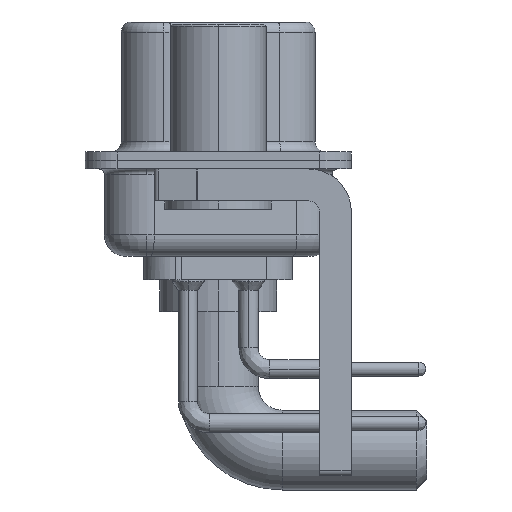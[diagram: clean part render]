
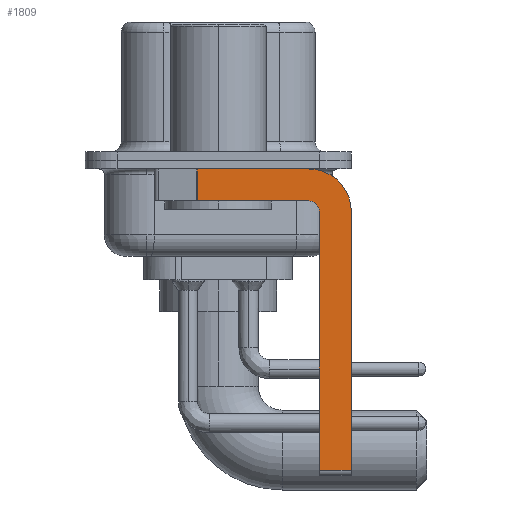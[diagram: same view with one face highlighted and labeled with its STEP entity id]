
A CAD part, left-side view. The second image highlights one B-rep face of the part: STEP entity #1809.
In plain terms, the highlighted planar face has unit normal (-1, 0, 0).
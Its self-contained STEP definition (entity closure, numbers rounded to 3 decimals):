
#289 = VERTEX_POINT ( 'NONE', #27104 ) ;
#622 = VECTOR ( 'NONE', #12479, 1000. ) ;
#795 = VERTEX_POINT ( 'NONE', #12686 ) ;
#1060 = AXIS2_PLACEMENT_3D ( 'NONE', #16492, #27981, #20971 ) ;
#1572 = FACE_OUTER_BOUND ( 'NONE', #23255, .T. ) ;
#1809 = ADVANCED_FACE ( 'NONE', ( #1572 ), #20848, .F. ) ;
#2685 = AXIS2_PLACEMENT_3D ( 'NONE', #13749, #20355, #11168 ) ;
#2969 = EDGE_CURVE ( 'NONE', #4347, #5563, #23773, .T. ) ;
#3414 = VERTEX_POINT ( 'NONE', #17682 ) ;
#3593 = CARTESIAN_POINT ( 'NONE',  ( -2.9, -4.25, -0.4 ) ) ;
#4347 = VERTEX_POINT ( 'NONE', #28086 ) ;
#5406 = CARTESIAN_POINT ( 'NONE',  ( -2.9, -4.75, -14.8 ) ) ;
#5563 = VERTEX_POINT ( 'NONE', #19250 ) ;
#5698 = CARTESIAN_POINT ( 'NONE',  ( -2.9, -4.25, -1.9 ) ) ;
#6378 = LINE ( 'NONE', #10550, #23307 ) ;
#6904 = CARTESIAN_POINT ( 'NONE',  ( -2.9, -4.25, -1.9 ) ) ;
#7136 = EDGE_CURVE ( 'NONE', #10527, #289, #20111, .T. ) ;
#7400 = AXIS2_PLACEMENT_3D ( 'NONE', #25423, #16377, #23000 ) ;
#7750 = LINE ( 'NONE', #18804, #622 ) ;
#8350 = DIRECTION ( 'NONE',  ( 0., -1., 0. ) ) ;
#8371 = ORIENTED_EDGE ( 'NONE', *, *, #26813, .T. ) ;
#9350 = DIRECTION ( 'NONE',  ( 0., 1., 0. ) ) ;
#10527 = VERTEX_POINT ( 'NONE', #5698 ) ;
#10550 = CARTESIAN_POINT ( 'NONE',  ( -2.9, 0.978, -1.9 ) ) ;
#11168 = DIRECTION ( 'NONE',  ( 0., 0., 1. ) ) ;
#11460 = ORIENTED_EDGE ( 'NONE', *, *, #11891, .F. ) ;
#11857 = EDGE_CURVE ( 'NONE', #21754, #4347, #20358, .T. ) ;
#11891 = EDGE_CURVE ( 'NONE', #3414, #21754, #7750, .T. ) ;
#12121 = VECTOR ( 'NONE', #8350, 1000. ) ;
#12479 = DIRECTION ( 'NONE',  ( 0., -1., 0. ) ) ;
#12640 = VECTOR ( 'NONE', #16039, 1000. ) ;
#12686 = CARTESIAN_POINT ( 'NONE',  ( -2.9, -4.75, -2.4 ) ) ;
#12715 = EDGE_CURVE ( 'NONE', #25160, #5563, #14804, .T. ) ;
#12758 = ORIENTED_EDGE ( 'NONE', *, *, #18714, .F. ) ;
#12789 = CARTESIAN_POINT ( 'NONE',  ( -2.9, -4.25, -14.55 ) ) ;
#13749 = CARTESIAN_POINT ( 'NONE',  ( -2.9, -4.25, -2.4 ) ) ;
#14804 = LINE ( 'NONE', #12789, #12121 ) ;
#14861 = DIRECTION ( 'NONE',  ( 0., 0., -1. ) ) ;
#15983 = CIRCLE ( 'NONE', #2685, 0.5 ) ;
#16039 = DIRECTION ( 'NONE',  ( 0., 0., 1. ) ) ;
#16377 = DIRECTION ( 'NONE',  ( 1., 0., 0. ) ) ;
#16492 = CARTESIAN_POINT ( 'NONE',  ( -2.9, -4.25, -2.4 ) ) ;
#17517 = VECTOR ( 'NONE', #21772, 1000. ) ;
#17682 = CARTESIAN_POINT ( 'NONE',  ( -2.9, 0.978, -0.4 ) ) ;
#17866 = ORIENTED_EDGE ( 'NONE', *, *, #11857, .F. ) ;
#18714 = EDGE_CURVE ( 'NONE', #25160, #795, #25075, .T. ) ;
#18804 = CARTESIAN_POINT ( 'NONE',  ( -2.9, 3., -0.4 ) ) ;
#19250 = CARTESIAN_POINT ( 'NONE',  ( -2.9, -6.25, -14.55 ) ) ;
#19622 = CARTESIAN_POINT ( 'NONE',  ( -2.9, -6.25, -2.4 ) ) ;
#20111 = LINE ( 'NONE', #6904, #23884 ) ;
#20237 = CARTESIAN_POINT ( 'NONE',  ( -2.9, -4.75, -14.55 ) ) ;
#20355 = DIRECTION ( 'NONE',  ( -1., 0., 0. ) ) ;
#20358 = CIRCLE ( 'NONE', #1060, 2. ) ;
#20848 = PLANE ( 'NONE',  #7400 ) ;
#20971 = DIRECTION ( 'NONE',  ( 0., 0., -1. ) ) ;
#21754 = VERTEX_POINT ( 'NONE', #3593 ) ;
#21772 = DIRECTION ( 'NONE',  ( 0., 0., -1. ) ) ;
#22772 = ORIENTED_EDGE ( 'NONE', *, *, #27979, .F. ) ;
#23000 = DIRECTION ( 'NONE',  ( 0., 0., -1. ) ) ;
#23255 = EDGE_LOOP ( 'NONE', ( #11460, #8371, #26242, #22772, #12758, #25396, #27537, #17866 ) ) ;
#23307 = VECTOR ( 'NONE', #14861, 1000. ) ;
#23773 = LINE ( 'NONE', #19622, #17517 ) ;
#23884 = VECTOR ( 'NONE', #9350, 1000. ) ;
#25075 = LINE ( 'NONE', #5406, #12640 ) ;
#25160 = VERTEX_POINT ( 'NONE', #20237 ) ;
#25396 = ORIENTED_EDGE ( 'NONE', *, *, #12715, .T. ) ;
#25423 = CARTESIAN_POINT ( 'NONE',  ( -2.9, -4.25, -2.4 ) ) ;
#26242 = ORIENTED_EDGE ( 'NONE', *, *, #7136, .F. ) ;
#26813 = EDGE_CURVE ( 'NONE', #3414, #289, #6378, .T. ) ;
#27104 = CARTESIAN_POINT ( 'NONE',  ( -2.9, 0.978, -1.9 ) ) ;
#27537 = ORIENTED_EDGE ( 'NONE', *, *, #2969, .F. ) ;
#27979 = EDGE_CURVE ( 'NONE', #795, #10527, #15983, .T. ) ;
#27981 = DIRECTION ( 'NONE',  ( 1., 0., 0. ) ) ;
#28086 = CARTESIAN_POINT ( 'NONE',  ( -2.9, -6.25, -2.4 ) ) ;
